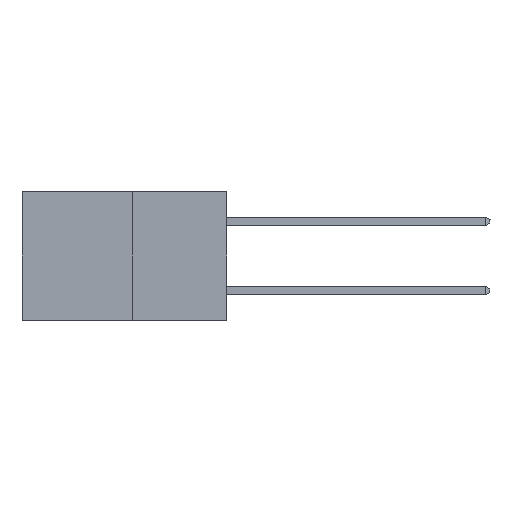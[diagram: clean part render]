
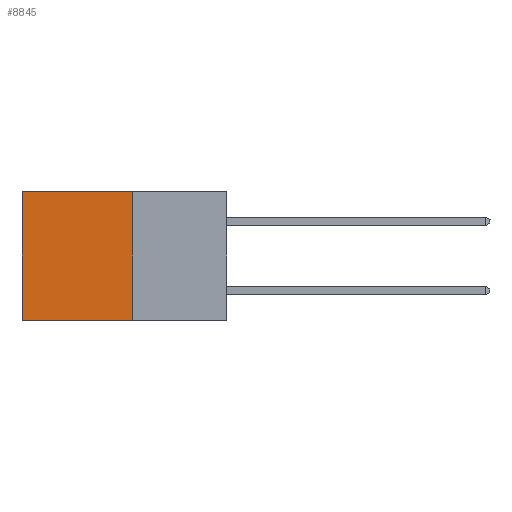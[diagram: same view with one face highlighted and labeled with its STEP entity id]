
A CAD part, left-side view. The second image highlights one B-rep face of the part: STEP entity #8845.
In plain terms, the highlighted planar face has unit normal (-1, 0, 0).
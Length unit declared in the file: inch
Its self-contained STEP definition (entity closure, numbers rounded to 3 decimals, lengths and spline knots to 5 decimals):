
#215 = CARTESIAN_POINT ( 'NONE',  ( 0.277, 0.27, -0.37 ) ) ;
#1378 = LINE ( 'NONE', #15461, #8154 ) ;
#1611 = VECTOR ( 'NONE', #3080, 39.37008 ) ;
#1806 = DIRECTION ( 'NONE',  ( 0., 1., 0. ) ) ;
#1835 = EDGE_CURVE ( 'NONE', #3848, #4701, #12183, .T. ) ;
#2107 = DIRECTION ( 'NONE',  ( 0., 1., 0. ) ) ;
#2310 = ORIENTED_EDGE ( 'NONE', *, *, #3951, .T. ) ;
#3002 = CARTESIAN_POINT ( 'NONE',  ( 0.277, 0.27, -0.37 ) ) ;
#3080 = DIRECTION ( 'NONE',  ( 0., 0., -1. ) ) ;
#3541 = AXIS2_PLACEMENT_3D ( 'NONE', #215, #5286, #9134 ) ;
#3595 = CARTESIAN_POINT ( 'NONE',  ( 0.277, 0.27, -0.37 ) ) ;
#3774 = DIRECTION ( 'NONE',  ( 0., 0., -1. ) ) ;
#3828 = CARTESIAN_POINT ( 'NONE',  ( 0.277, 0.59, 0. ) ) ;
#3848 = VERTEX_POINT ( 'NONE', #11116 ) ;
#3951 = EDGE_CURVE ( 'NONE', #4701, #5457, #12306, .T. ) ;
#4496 = EDGE_CURVE ( 'NONE', #9262, #5457, #1378, .T. ) ;
#4701 = VERTEX_POINT ( 'NONE', #3828 ) ;
#5268 = PLANE ( 'NONE',  #3541 ) ;
#5286 = DIRECTION ( 'NONE',  ( 1., 0., 0. ) ) ;
#5457 = VERTEX_POINT ( 'NONE', #13155 ) ;
#7794 = EDGE_CURVE ( 'NONE', #3848, #9262, #11756, .T. ) ;
#7898 = EDGE_LOOP ( 'NONE', ( #2310, #15907, #12781, #9922 ) ) ;
#8154 = VECTOR ( 'NONE', #1806, 39.37008 ) ;
#8845 = ADVANCED_FACE ( 'NONE', ( #10176 ), #5268, .F. ) ;
#9134 = DIRECTION ( 'NONE',  ( 0., 0., -1. ) ) ;
#9262 = VERTEX_POINT ( 'NONE', #3595 ) ;
#9922 = ORIENTED_EDGE ( 'NONE', *, *, #1835, .T. ) ;
#10176 = FACE_OUTER_BOUND ( 'NONE', #7898, .T. ) ;
#10515 = CARTESIAN_POINT ( 'NONE',  ( 0.277, 0.27, 0. ) ) ;
#11116 = CARTESIAN_POINT ( 'NONE',  ( 0.277, 0.27, 0. ) ) ;
#11756 = LINE ( 'NONE', #3002, #1611 ) ;
#11807 = VECTOR ( 'NONE', #2107, 39.37008 ) ;
#12183 = LINE ( 'NONE', #10515, #11807 ) ;
#12306 = LINE ( 'NONE', #15800, #15449 ) ;
#12781 = ORIENTED_EDGE ( 'NONE', *, *, #7794, .F. ) ;
#13155 = CARTESIAN_POINT ( 'NONE',  ( 0.277, 0.59, -0.37 ) ) ;
#15449 = VECTOR ( 'NONE', #3774, 39.37008 ) ;
#15461 = CARTESIAN_POINT ( 'NONE',  ( 0.277, 0.27, -0.37 ) ) ;
#15800 = CARTESIAN_POINT ( 'NONE',  ( 0.277, 0.59, -0.37 ) ) ;
#15907 = ORIENTED_EDGE ( 'NONE', *, *, #4496, .F. ) ;
